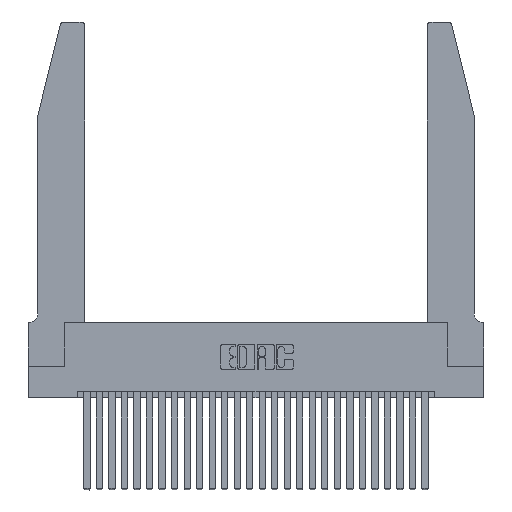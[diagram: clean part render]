
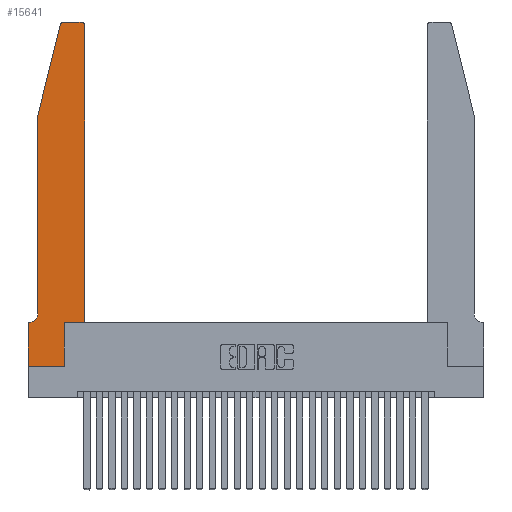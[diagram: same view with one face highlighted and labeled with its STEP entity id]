
A CAD part, top view. The second image highlights one B-rep face of the part: STEP entity #15641.
In plain terms, the highlighted planar face has unit normal (0, 0, 1).
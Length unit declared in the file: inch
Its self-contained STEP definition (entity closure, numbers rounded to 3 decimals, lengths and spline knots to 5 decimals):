
#535 = ORIENTED_EDGE ( 'NONE', *, *, #14381, .T. ) ;
#603 = DIRECTION ( 'NONE',  ( -1., 0., 0. ) ) ;
#1562 = CARTESIAN_POINT ( 'NONE',  ( 0.284, 2.75, 0.37 ) ) ;
#1644 = CARTESIAN_POINT ( 'NONE',  ( 0.25487, 2.72718, 0.37 ) ) ;
#2172 = DIRECTION ( 'NONE',  ( 0., 0., 1. ) ) ;
#2179 = ORIENTED_EDGE ( 'NONE', *, *, #28189, .T. ) ;
#2465 = DIRECTION ( 'NONE',  ( 1., 0., 0. ) ) ;
#2507 = CARTESIAN_POINT ( 'NONE',  ( 0., 0.35, 0.37 ) ) ;
#2926 = EDGE_CURVE ( 'NONE', #20985, #12698, #24998, .T. ) ;
#3038 = CIRCLE ( 'NONE', #24878, 0.07 ) ;
#3059 = ORIENTED_EDGE ( 'NONE', *, *, #3094, .T. ) ;
#3094 = EDGE_CURVE ( 'NONE', #27149, #12491, #15654, .T. ) ;
#3494 = DIRECTION ( 'NONE',  ( 1., 0., 0. ) ) ;
#3771 = CARTESIAN_POINT ( 'NONE',  ( 0., 0., 0.37 ) ) ;
#3804 = DIRECTION ( 'NONE',  ( 0., -1., 0. ) ) ;
#3944 = ORIENTED_EDGE ( 'NONE', *, *, #16650, .T. ) ;
#4980 = VERTEX_POINT ( 'NONE', #8670 ) ;
#5931 = CARTESIAN_POINT ( 'NONE',  ( 0.4505, 2.72, 0.37 ) ) ;
#6305 = VERTEX_POINT ( 'NONE', #23336 ) ;
#6729 = ORIENTED_EDGE ( 'NONE', *, *, #25626, .T. ) ;
#6770 = VECTOR ( 'NONE', #23836, 39.37008 ) ;
#6840 = VERTEX_POINT ( 'NONE', #20564 ) ;
#6984 = LINE ( 'NONE', #21802, #16963 ) ;
#7951 = CARTESIAN_POINT ( 'NONE',  ( 0., 0., 0.37 ) ) ;
#8047 = PLANE ( 'NONE',  #14600 ) ;
#8670 = CARTESIAN_POINT ( 'NONE',  ( 0.0755, 2., 0.37 ) ) ;
#8865 = EDGE_CURVE ( 'NONE', #6305, #11430, #3038, .T. ) ;
#9107 = FACE_OUTER_BOUND ( 'NONE', #14160, .T. ) ;
#9291 = VERTEX_POINT ( 'NONE', #2507 ) ;
#9471 = CARTESIAN_POINT ( 'NONE',  ( 0.2605, 2.75, 0.37 ) ) ;
#10502 = ORIENTED_EDGE ( 'NONE', *, *, #13239, .T. ) ;
#10833 = VERTEX_POINT ( 'NONE', #1644 ) ;
#11004 = CIRCLE ( 'NONE', #24348, 0.03 ) ;
#11430 = VERTEX_POINT ( 'NONE', #14816 ) ;
#11680 = CARTESIAN_POINT ( 'NONE',  ( 0.0055, 0.42, 0.37 ) ) ;
#11721 = EDGE_CURVE ( 'NONE', #12491, #24774, #16906, .T. ) ;
#12222 = VERTEX_POINT ( 'NONE', #26889 ) ;
#12491 = VERTEX_POINT ( 'NONE', #12886 ) ;
#12568 = CARTESIAN_POINT ( 'NONE',  ( 0.0755, 0.35, 0.37 ) ) ;
#12572 = DIRECTION ( 'NONE',  ( 0., 0., 1. ) ) ;
#12698 = VERTEX_POINT ( 'NONE', #26837 ) ;
#12886 = CARTESIAN_POINT ( 'NONE',  ( 0.4205, 2.75, 0.37 ) ) ;
#13054 = LINE ( 'NONE', #20485, #16540 ) ;
#13239 = EDGE_CURVE ( 'NONE', #6840, #27149, #13054, .T. ) ;
#13740 = ORIENTED_EDGE ( 'NONE', *, *, #22959, .T. ) ;
#14160 = EDGE_LOOP ( 'NONE', ( #18475, #6729, #21564, #13740, #21301, #2179, #24087, #24186, #535, #3944, #10502, #3059 ) ) ;
#14381 = EDGE_CURVE ( 'NONE', #12698, #12222, #25453, .T. ) ;
#14600 = AXIS2_PLACEMENT_3D ( 'NONE', #16918, #12572, #3494 ) ;
#14816 = CARTESIAN_POINT ( 'NONE',  ( 0.0055, 0.35, 0.37 ) ) ;
#15305 = CARTESIAN_POINT ( 'NONE',  ( 0.284, 2.72, 0.37 ) ) ;
#15641 = ADVANCED_FACE ( 'NONE', ( #9107 ), #8047, .T. ) ;
#15654 = CIRCLE ( 'NONE', #22383, 0.03 ) ;
#15929 = DIRECTION ( 'NONE',  ( 0., 0., -1. ) ) ;
#16113 = CARTESIAN_POINT ( 'NONE',  ( 0.0755, 2., 0.37 ) ) ;
#16540 = VECTOR ( 'NONE', #26989, 39.37008 ) ;
#16650 = EDGE_CURVE ( 'NONE', #12222, #6840, #17702, .T. ) ;
#16906 = LINE ( 'NONE', #9471, #18315 ) ;
#16918 = CARTESIAN_POINT ( 'NONE',  ( 0., 0.35, 0.37 ) ) ;
#16934 = CARTESIAN_POINT ( 'NONE',  ( 0.2865, 0.35, 0.37 ) ) ;
#16963 = VECTOR ( 'NONE', #3804, 39.37008 ) ;
#17702 = LINE ( 'NONE', #26392, #28350 ) ;
#18164 = EDGE_CURVE ( 'NONE', #10833, #4980, #23456, .T. ) ;
#18315 = VECTOR ( 'NONE', #603, 39.37008 ) ;
#18475 = ORIENTED_EDGE ( 'NONE', *, *, #11721, .T. ) ;
#18586 = DIRECTION ( 'NONE',  ( 0., 0., 1. ) ) ;
#20485 = CARTESIAN_POINT ( 'NONE',  ( 0.4505, 0.35, 0.37 ) ) ;
#20564 = CARTESIAN_POINT ( 'NONE',  ( 0.4505, 0.35, 0.37 ) ) ;
#20961 = VECTOR ( 'NONE', #24060, 39.37008 ) ;
#20985 = VERTEX_POINT ( 'NONE', #7951 ) ;
#21301 = ORIENTED_EDGE ( 'NONE', *, *, #8865, .T. ) ;
#21564 = ORIENTED_EDGE ( 'NONE', *, *, #18164, .T. ) ;
#21802 = CARTESIAN_POINT ( 'NONE',  ( 0., 0., 0.37 ) ) ;
#22383 = AXIS2_PLACEMENT_3D ( 'NONE', #27196, #18586, #24817 ) ;
#22959 = EDGE_CURVE ( 'NONE', #4980, #6305, #26928, .T. ) ;
#23336 = CARTESIAN_POINT ( 'NONE',  ( 0.0755, 0.42, 0.37 ) ) ;
#23456 = LINE ( 'NONE', #16113, #27886 ) ;
#23681 = CARTESIAN_POINT ( 'NONE',  ( 0.0755, 2., 0.37 ) ) ;
#23836 = DIRECTION ( 'NONE',  ( -1., 0., 0. ) ) ;
#24060 = DIRECTION ( 'NONE',  ( 0., 1., 0. ) ) ;
#24087 = ORIENTED_EDGE ( 'NONE', *, *, #24223, .T. ) ;
#24186 = ORIENTED_EDGE ( 'NONE', *, *, #2926, .T. ) ;
#24223 = EDGE_CURVE ( 'NONE', #9291, #20985, #6984, .T. ) ;
#24348 = AXIS2_PLACEMENT_3D ( 'NONE', #15305, #2172, #2465 ) ;
#24528 = VECTOR ( 'NONE', #27986, 39.37008 ) ;
#24774 = VERTEX_POINT ( 'NONE', #1562 ) ;
#24817 = DIRECTION ( 'NONE',  ( 1., 0., 0. ) ) ;
#24878 = AXIS2_PLACEMENT_3D ( 'NONE', #11680, #15929, #27280 ) ;
#24998 = LINE ( 'NONE', #3771, #25672 ) ;
#25453 = LINE ( 'NONE', #16934, #20961 ) ;
#25626 = EDGE_CURVE ( 'NONE', #24774, #10833, #11004, .T. ) ;
#25672 = VECTOR ( 'NONE', #27975, 39.37008 ) ;
#26392 = CARTESIAN_POINT ( 'NONE',  ( 0.4505, 0.35, 0.37 ) ) ;
#26767 = DIRECTION ( 'NONE',  ( 1., 0., 0. ) ) ;
#26837 = CARTESIAN_POINT ( 'NONE',  ( 0.2865, 0., 0.37 ) ) ;
#26889 = CARTESIAN_POINT ( 'NONE',  ( 0.2865, 0.35, 0.37 ) ) ;
#26928 = LINE ( 'NONE', #23681, #24528 ) ;
#26989 = DIRECTION ( 'NONE',  ( 0., 1., 0. ) ) ;
#27149 = VERTEX_POINT ( 'NONE', #5931 ) ;
#27196 = CARTESIAN_POINT ( 'NONE',  ( 0.4205, 2.72, 0.37 ) ) ;
#27273 = DIRECTION ( 'NONE',  ( -0.239, -0.971, 0. ) ) ;
#27280 = DIRECTION ( 'NONE',  ( -1., 0., 0. ) ) ;
#27761 = LINE ( 'NONE', #12568, #6770 ) ;
#27886 = VECTOR ( 'NONE', #27273, 39.37008 ) ;
#27975 = DIRECTION ( 'NONE',  ( 1., 0., 0. ) ) ;
#27986 = DIRECTION ( 'NONE',  ( 0., -1., 0. ) ) ;
#28189 = EDGE_CURVE ( 'NONE', #11430, #9291, #27761, .T. ) ;
#28350 = VECTOR ( 'NONE', #26767, 39.37008 ) ;
